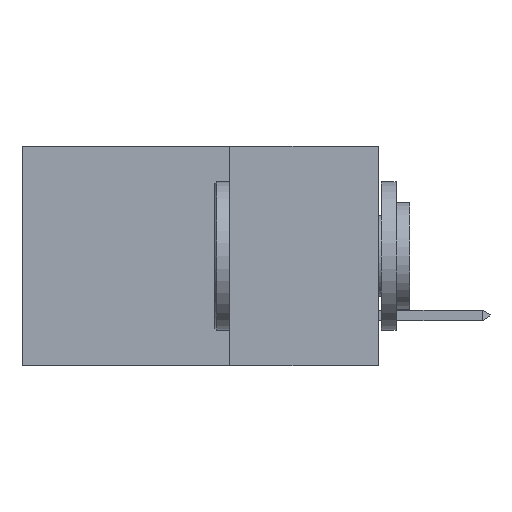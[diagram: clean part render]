
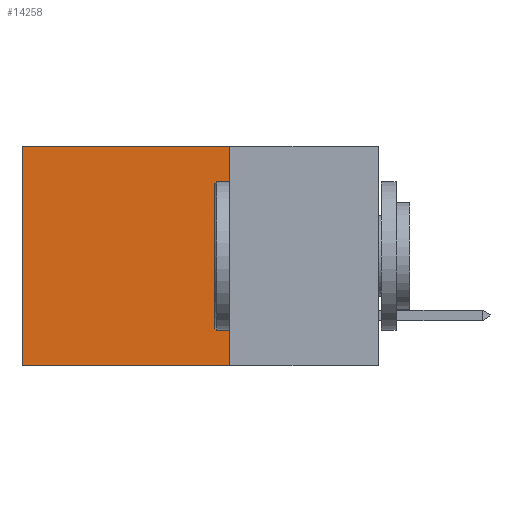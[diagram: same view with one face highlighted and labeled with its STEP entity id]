
A CAD part, left-side view. The second image highlights one B-rep face of the part: STEP entity #14258.
In plain terms, the highlighted planar face has unit normal (-1, 0, 0).
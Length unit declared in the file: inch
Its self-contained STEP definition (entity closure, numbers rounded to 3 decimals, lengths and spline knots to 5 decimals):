
#89 = CARTESIAN_POINT ( 'NONE',  ( 0.298, 0.6, -0.37 ) ) ;
#166 = VECTOR ( 'NONE', #23329, 39.37008 ) ;
#282 = VERTEX_POINT ( 'NONE', #4458 ) ;
#508 = LINE ( 'NONE', #1956, #10329 ) ;
#815 = DIRECTION ( 'NONE',  ( 0., 0., -1. ) ) ;
#1956 = CARTESIAN_POINT ( 'NONE',  ( 0.298, 0.25, 0. ) ) ;
#2157 = LINE ( 'NONE', #3728, #7502 ) ;
#2411 = FACE_OUTER_BOUND ( 'NONE', #6920, .T. ) ;
#2470 = VERTEX_POINT ( 'NONE', #89 ) ;
#3413 = DIRECTION ( 'NONE',  ( 0., 0., -1. ) ) ;
#3728 = CARTESIAN_POINT ( 'NONE',  ( 0.298, 0.6, 0. ) ) ;
#4458 = CARTESIAN_POINT ( 'NONE',  ( 0.298, 0.25, 0. ) ) ;
#5211 = LINE ( 'NONE', #17850, #166 ) ;
#5466 = ORIENTED_EDGE ( 'NONE', *, *, #22013, .T. ) ;
#6149 = VECTOR ( 'NONE', #10505, 39.37008 ) ;
#6920 = EDGE_LOOP ( 'NONE', ( #23132, #8975, #22897, #5466 ) ) ;
#7502 = VECTOR ( 'NONE', #3413, 39.37008 ) ;
#8975 = ORIENTED_EDGE ( 'NONE', *, *, #20274, .F. ) ;
#9994 = PLANE ( 'NONE',  #16378 ) ;
#10098 = VERTEX_POINT ( 'NONE', #17788 ) ;
#10329 = VECTOR ( 'NONE', #17269, 39.37008 ) ;
#10505 = DIRECTION ( 'NONE',  ( 0., 1., 0. ) ) ;
#10595 = CARTESIAN_POINT ( 'NONE',  ( 0.298, 0.25, 0. ) ) ;
#10638 = LINE ( 'NONE', #10595, #6149 ) ;
#11840 = CARTESIAN_POINT ( 'NONE',  ( 0.298, 0.25, 0. ) ) ;
#11903 = CARTESIAN_POINT ( 'NONE',  ( 0.298, 0.6, 0. ) ) ;
#14258 = ADVANCED_FACE ( 'NONE', ( #2411 ), #9994, .F. ) ;
#15629 = EDGE_CURVE ( 'NONE', #17415, #2470, #2157, .T. ) ;
#16221 = DIRECTION ( 'NONE',  ( 1., 0., 0. ) ) ;
#16378 = AXIS2_PLACEMENT_3D ( 'NONE', #11840, #16221, #815 ) ;
#17269 = DIRECTION ( 'NONE',  ( 0., 0., -1. ) ) ;
#17415 = VERTEX_POINT ( 'NONE', #11903 ) ;
#17788 = CARTESIAN_POINT ( 'NONE',  ( 0.298, 0.25, -0.37 ) ) ;
#17850 = CARTESIAN_POINT ( 'NONE',  ( 0.298, 0.25, -0.37 ) ) ;
#19067 = EDGE_CURVE ( 'NONE', #282, #10098, #508, .T. ) ;
#20274 = EDGE_CURVE ( 'NONE', #10098, #2470, #5211, .T. ) ;
#22013 = EDGE_CURVE ( 'NONE', #282, #17415, #10638, .T. ) ;
#22897 = ORIENTED_EDGE ( 'NONE', *, *, #19067, .F. ) ;
#23132 = ORIENTED_EDGE ( 'NONE', *, *, #15629, .T. ) ;
#23329 = DIRECTION ( 'NONE',  ( 0., 1., 0. ) ) ;
